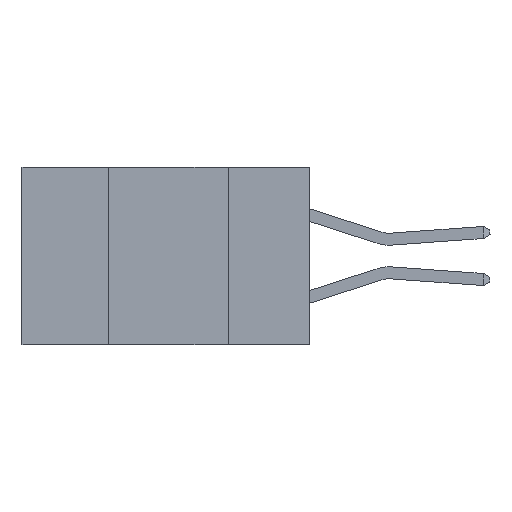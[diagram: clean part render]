
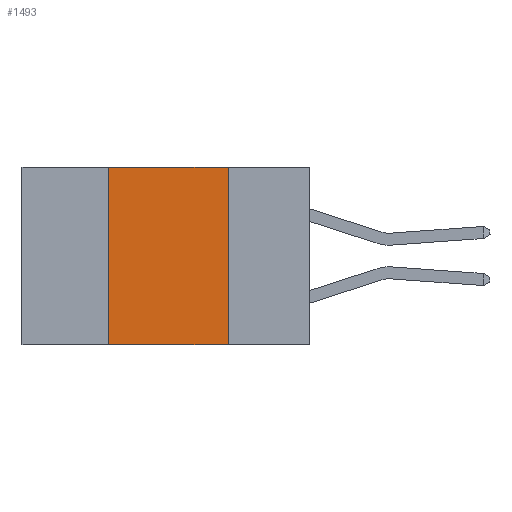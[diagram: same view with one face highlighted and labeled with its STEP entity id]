
A CAD part, left-side view. The second image highlights one B-rep face of the part: STEP entity #1493.
In plain terms, the highlighted planar face has unit normal (-1, 0, 0).
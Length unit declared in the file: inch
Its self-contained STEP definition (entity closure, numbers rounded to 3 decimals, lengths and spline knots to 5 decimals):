
#137 = LINE ( 'NONE', #893, #2610 ) ;
#265 = EDGE_CURVE ( 'NONE', #4475, #11035, #2557, .T. ) ;
#893 = CARTESIAN_POINT ( 'NONE',  ( 0., 0.17, -0.37 ) ) ;
#996 = DIRECTION ( 'NONE',  ( 0., 0., -1. ) ) ;
#1493 = ADVANCED_FACE ( 'NONE', ( #4145 ), #3398, .F. ) ;
#1862 = VECTOR ( 'NONE', #4039, 39.37008 ) ;
#1887 = ORIENTED_EDGE ( 'NONE', *, *, #5775, .F. ) ;
#2135 = VECTOR ( 'NONE', #8898, 39.37008 ) ;
#2151 = DIRECTION ( 'NONE',  ( 0., 0., -1. ) ) ;
#2197 = LINE ( 'NONE', #4061, #1862 ) ;
#2417 = CARTESIAN_POINT ( 'NONE',  ( 0., 0.42, -0.37 ) ) ;
#2474 = DIRECTION ( 'NONE',  ( 1., 0., 0. ) ) ;
#2557 = LINE ( 'NONE', #3653, #10256 ) ;
#2610 = VECTOR ( 'NONE', #996, 39.37008 ) ;
#2627 = CARTESIAN_POINT ( 'NONE',  ( 0., 0.6, 0. ) ) ;
#3009 = CARTESIAN_POINT ( 'NONE',  ( 0., 0.42, 0. ) ) ;
#3398 = PLANE ( 'NONE',  #7911 ) ;
#3522 = EDGE_CURVE ( 'NONE', #4475, #11348, #7526, .T. ) ;
#3653 = CARTESIAN_POINT ( 'NONE',  ( 0., 0.6, -0.37 ) ) ;
#4039 = DIRECTION ( 'NONE',  ( 0., -1., 0. ) ) ;
#4061 = CARTESIAN_POINT ( 'NONE',  ( 0., 0.6, 0. ) ) ;
#4145 = FACE_OUTER_BOUND ( 'NONE', #4747, .T. ) ;
#4475 = VERTEX_POINT ( 'NONE', #2417 ) ;
#4747 = EDGE_LOOP ( 'NONE', ( #1887, #7592, #7907, #8234 ) ) ;
#5334 = DIRECTION ( 'NONE',  ( 0., -1., 0. ) ) ;
#5775 = EDGE_CURVE ( 'NONE', #6098, #11035, #137, .T. ) ;
#6098 = VERTEX_POINT ( 'NONE', #7163 ) ;
#7163 = CARTESIAN_POINT ( 'NONE',  ( 0., 0.17, 0. ) ) ;
#7526 = LINE ( 'NONE', #8813, #2135 ) ;
#7592 = ORIENTED_EDGE ( 'NONE', *, *, #9312, .F. ) ;
#7907 = ORIENTED_EDGE ( 'NONE', *, *, #3522, .F. ) ;
#7911 = AXIS2_PLACEMENT_3D ( 'NONE', #2627, #2474, #2151 ) ;
#8234 = ORIENTED_EDGE ( 'NONE', *, *, #265, .T. ) ;
#8813 = CARTESIAN_POINT ( 'NONE',  ( 0., 0.42, -0.37 ) ) ;
#8898 = DIRECTION ( 'NONE',  ( 0., 0., 1. ) ) ;
#9312 = EDGE_CURVE ( 'NONE', #11348, #6098, #2197, .T. ) ;
#9610 = CARTESIAN_POINT ( 'NONE',  ( 0., 0.17, -0.37 ) ) ;
#10256 = VECTOR ( 'NONE', #5334, 39.37008 ) ;
#11035 = VERTEX_POINT ( 'NONE', #9610 ) ;
#11348 = VERTEX_POINT ( 'NONE', #3009 ) ;
